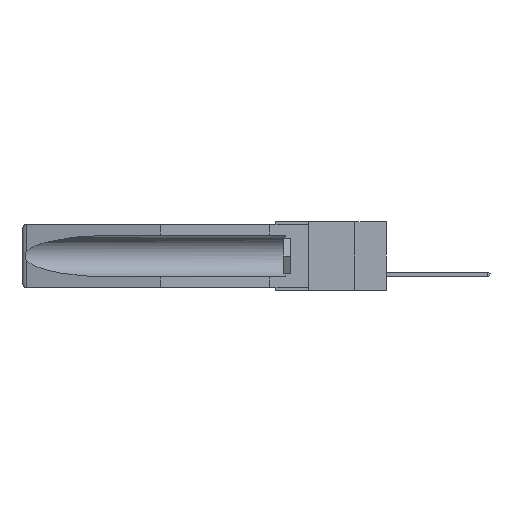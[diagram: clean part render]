
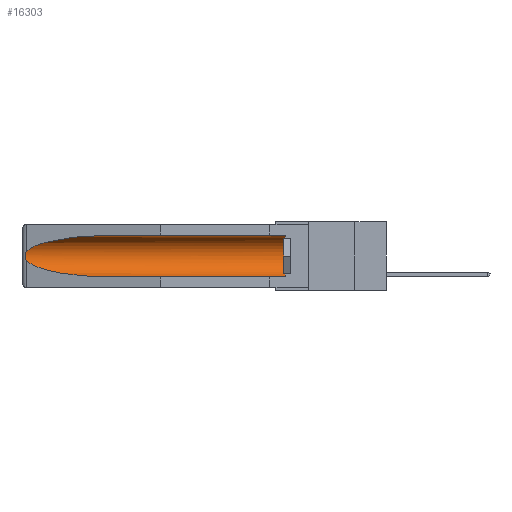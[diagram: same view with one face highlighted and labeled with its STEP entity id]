
A CAD part, left-side view. The second image highlights one B-rep face of the part: STEP entity #16303.
In plain terms, the highlighted cylindrical face has radius 2.857 mm (diameter 5.715 mm), a partial arc.
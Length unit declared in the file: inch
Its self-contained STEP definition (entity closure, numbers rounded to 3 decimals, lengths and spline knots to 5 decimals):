
#276 = VERTEX_POINT ( 'NONE', #10939 ) ;
#564 = CARTESIAN_POINT ( 'NONE',  ( 0.2675, 1.53308, -0.17534 ) ) ;
#575 = AXIS2_PLACEMENT_3D ( 'NONE', #10093, #5687, #5808 ) ;
#579 = VECTOR ( 'NONE', #14443, 39.37008 ) ;
#1819 = CARTESIAN_POINT ( 'NONE',  ( 0.26597, 1.52961, -0.15275 ) ) ;
#1940 = CARTESIAN_POINT ( 'NONE',  ( 0.26597, 1.5296, -0.19026 ) ) ;
#2023 = CYLINDRICAL_SURFACE ( 'NONE', #575, 0.1125 ) ;
#2084 = DIRECTION ( 'NONE',  ( 0., 1., 0. ) ) ;
#2214 = VERTEX_POINT ( 'NONE', #12154 ) ;
#2404 = CARTESIAN_POINT ( 'NONE',  ( 0.26537, 1.52718, -0.19328 ) ) ;
#2446 =( BOUNDED_CURVE ( )  B_SPLINE_CURVE ( 3, ( #12968, #11581, #3621, #15984 ),
 .UNSPECIFIED., .F., .F. ) 
 B_SPLINE_CURVE_WITH_KNOTS ( ( 4, 4 ),
 ( 0.1948, 1.5708 ),
 .UNSPECIFIED. ) 
 CURVE ( )  GEOMETRIC_REPRESENTATION_ITEM ( )  RATIONAL_B_SPLINE_CURVE ( ( 1., 0.848, 0.848, 1. ) ) 
 REPRESENTATION_ITEM ( '' )  );
#2462 = VERTEX_POINT ( 'NONE', #3091 ) ;
#2579 = ORIENTED_EDGE ( 'NONE', *, *, #4849, .T. ) ;
#3091 = CARTESIAN_POINT ( 'NONE',  ( 0.155, 1.07973, -0.284 ) ) ;
#3306 = ORIENTED_EDGE ( 'NONE', *, *, #8258, .T. ) ;
#3325 = CARTESIAN_POINT ( 'NONE',  ( 0.26537, 1.52718, -0.19328 ) ) ;
#3454 = CARTESIAN_POINT ( 'NONE',  ( 0.26537, 1.52718, -0.14972 ) ) ;
#3511 = CARTESIAN_POINT ( 'NONE',  ( 0.25451, 1.48313, -0.09465 ) ) ;
#3621 = CARTESIAN_POINT ( 'NONE',  ( 0.21114, 1.30732, -0.284 ) ) ;
#4046 = CARTESIAN_POINT ( 'NONE',  ( 0.155, 0.126, -0.1715 ) ) ;
#4505 = VERTEX_POINT ( 'NONE', #2404 ) ;
#4643 = CARTESIAN_POINT ( 'NONE',  ( 0.26654, 1.53092, -0.15636 ) ) ;
#4849 = EDGE_CURVE ( 'NONE', #276, #9671, #14139, .T. ) ;
#5687 = DIRECTION ( 'NONE',  ( 0., 1., 0. ) ) ;
#5808 = DIRECTION ( 'NONE',  ( 0., 0., 1. ) ) ;
#6398 = ORIENTED_EDGE ( 'NONE', *, *, #12617, .T. ) ;
#6801 = FACE_OUTER_BOUND ( 'NONE', #16929, .T. ) ;
#8258 = EDGE_CURVE ( 'NONE', #2214, #276, #10574, .T. ) ;
#9081 = CARTESIAN_POINT ( 'NONE',  ( 0.155, 1.07973, -0.059 ) ) ;
#9122 = CARTESIAN_POINT ( 'NONE',  ( 0.26537, 1.52718, -0.14972 ) ) ;
#9520 = EDGE_CURVE ( 'NONE', #2214, #2462, #17372, .T. ) ;
#9671 = VERTEX_POINT ( 'NONE', #13473 ) ;
#9843 = ORIENTED_EDGE ( 'NONE', *, *, #14725, .T. ) ;
#9996 = CARTESIAN_POINT ( 'NONE',  ( 0.155, -0.30754, -0.284 ) ) ;
#10093 = CARTESIAN_POINT ( 'NONE',  ( 0.155, -0.30754, -0.1715 ) ) ;
#10574 = CIRCLE ( 'NONE', #11439, 0.1125 ) ;
#10618 = CARTESIAN_POINT ( 'NONE',  ( 0.155, -0.30754, -0.059 ) ) ;
#10831 = ORIENTED_EDGE ( 'NONE', *, *, #9520, .F. ) ;
#10939 = CARTESIAN_POINT ( 'NONE',  ( 0.155, 0.126, -0.059 ) ) ;
#11439 = AXIS2_PLACEMENT_3D ( 'NONE', #4046, #15031, #14915 ) ;
#11581 = CARTESIAN_POINT ( 'NONE',  ( 0.25451, 1.48313, -0.24835 ) ) ;
#11582 = CARTESIAN_POINT ( 'NONE',  ( 0.26655, 1.53094, -0.18657 ) ) ;
#12154 = CARTESIAN_POINT ( 'NONE',  ( 0.155, 0.126, -0.284 ) ) ;
#12617 = EDGE_CURVE ( 'NONE', #9671, #13200, #14816, .T. ) ;
#12906 = CARTESIAN_POINT ( 'NONE',  ( 0.26537, 1.52718, -0.14972 ) ) ;
#12968 = CARTESIAN_POINT ( 'NONE',  ( 0.26537, 1.52718, -0.19328 ) ) ;
#12984 = CARTESIAN_POINT ( 'NONE',  ( 0.21114, 1.30732, -0.059 ) ) ;
#13067 = EDGE_CURVE ( 'NONE', #13200, #4505, #13165, .T. ) ;
#13165 = B_SPLINE_CURVE_WITH_KNOTS ( 'NONE', 3,
 ( #12906, #1819, #4643, #15679, #17062, #564, #14053, #11582, #1940, #3325 ),
 .UNSPECIFIED., .F., .F.,
 ( 4, 2, 2, 2, 4 ),
 ( 0., 0.00029, 0.00058, 0.00087, 0.00117 ),
 .UNSPECIFIED. ) ;
#13200 = VERTEX_POINT ( 'NONE', #9122 ) ;
#13473 = CARTESIAN_POINT ( 'NONE',  ( 0.155, 1.07973, -0.059 ) ) ;
#13715 = VECTOR ( 'NONE', #2084, 39.37008 ) ;
#14053 = CARTESIAN_POINT ( 'NONE',  ( 0.2673, 1.53269, -0.17917 ) ) ;
#14139 = LINE ( 'NONE', #10618, #579 ) ;
#14443 = DIRECTION ( 'NONE',  ( 0., 1., 0. ) ) ;
#14725 = EDGE_CURVE ( 'NONE', #4505, #2462, #2446, .T. ) ;
#14816 =( BOUNDED_CURVE ( )  B_SPLINE_CURVE ( 3, ( #9081, #12984, #3511, #3454 ),
 .UNSPECIFIED., .F., .F. ) 
 B_SPLINE_CURVE_WITH_KNOTS ( ( 4, 4 ),
 ( 4.71239, 6.08839 ),
 .UNSPECIFIED. ) 
 CURVE ( )  GEOMETRIC_REPRESENTATION_ITEM ( )  RATIONAL_B_SPLINE_CURVE ( ( 1., 0.848, 0.848, 1. ) ) 
 REPRESENTATION_ITEM ( '' )  );
#14915 = DIRECTION ( 'NONE',  ( 0., 0., 1. ) ) ;
#15031 = DIRECTION ( 'NONE',  ( 0., -1., 0. ) ) ;
#15679 = CARTESIAN_POINT ( 'NONE',  ( 0.2673, 1.5327, -0.16383 ) ) ;
#15984 = CARTESIAN_POINT ( 'NONE',  ( 0.155, 1.07973, -0.284 ) ) ;
#16303 = ADVANCED_FACE ( 'NONE', ( #6801 ), #2023, .F. ) ;
#16881 = ORIENTED_EDGE ( 'NONE', *, *, #13067, .T. ) ;
#16929 = EDGE_LOOP ( 'NONE', ( #6398, #16881, #9843, #10831, #3306, #2579 ) ) ;
#17062 = CARTESIAN_POINT ( 'NONE',  ( 0.2675, 1.53308, -0.16763 ) ) ;
#17372 = LINE ( 'NONE', #9996, #13715 ) ;
